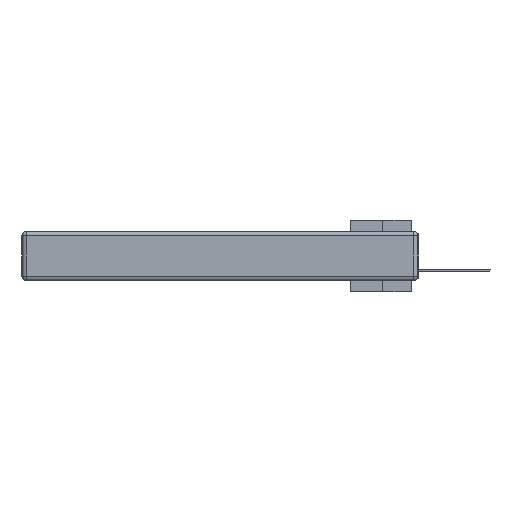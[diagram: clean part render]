
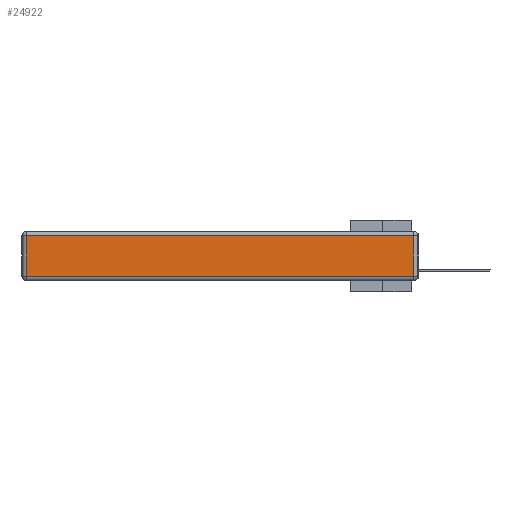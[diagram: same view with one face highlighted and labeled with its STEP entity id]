
A CAD part, left-side view. The second image highlights one B-rep face of the part: STEP entity #24922.
In plain terms, the highlighted planar face has unit normal (-1, 0, 0).
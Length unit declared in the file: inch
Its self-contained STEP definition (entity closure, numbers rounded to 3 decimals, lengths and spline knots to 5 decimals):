
#3186 = VERTEX_POINT ( 'NONE', #13487 ) ;
#3708 = DIRECTION ( 'NONE',  ( 0., 0., 1. ) ) ;
#5612 = EDGE_CURVE ( 'NONE', #34793, #3186, #30370, .T. ) ;
#5786 = EDGE_CURVE ( 'NONE', #8883, #22546, #15652, .T. ) ;
#5871 = CARTESIAN_POINT ( 'NONE',  ( 0., 2.72, -0.313 ) ) ;
#8045 = CARTESIAN_POINT ( 'NONE',  ( 0., 2.75, -0.03 ) ) ;
#8883 = VERTEX_POINT ( 'NONE', #5871 ) ;
#9691 = LINE ( 'NONE', #19569, #11995 ) ;
#11995 = VECTOR ( 'NONE', #25467, 39.37008 ) ;
#12415 = CARTESIAN_POINT ( 'NONE',  ( 0., 0., -0.343 ) ) ;
#13423 = FACE_OUTER_BOUND ( 'NONE', #18129, .T. ) ;
#13487 = CARTESIAN_POINT ( 'NONE',  ( 0., 2.72, -0.03 ) ) ;
#13542 = ORIENTED_EDGE ( 'NONE', *, *, #23218, .T. ) ;
#14140 = ORIENTED_EDGE ( 'NONE', *, *, #5786, .T. ) ;
#14721 = DIRECTION ( 'NONE',  ( 0., -1., 0. ) ) ;
#15652 = LINE ( 'NONE', #29110, #27167 ) ;
#18129 = EDGE_LOOP ( 'NONE', ( #14140, #28127, #31392, #13542 ) ) ;
#18329 = DIRECTION ( 'NONE',  ( -1., 0., 0. ) ) ;
#19569 = CARTESIAN_POINT ( 'NONE',  ( 0., 0.03, -0.343 ) ) ;
#21545 = CARTESIAN_POINT ( 'NONE',  ( 0., 0.03, -0.313 ) ) ;
#21897 = DIRECTION ( 'NONE',  ( 0., 0., -1. ) ) ;
#22546 = VERTEX_POINT ( 'NONE', #21545 ) ;
#23218 = EDGE_CURVE ( 'NONE', #3186, #8883, #34730, .T. ) ;
#24922 = ADVANCED_FACE ( 'NONE', ( #13423 ), #30014, .T. ) ;
#25467 = DIRECTION ( 'NONE',  ( 0., 0., 1. ) ) ;
#25581 = EDGE_CURVE ( 'NONE', #22546, #34793, #9691, .T. ) ;
#26305 = CARTESIAN_POINT ( 'NONE',  ( 0., 0.03, -0.03 ) ) ;
#26621 = AXIS2_PLACEMENT_3D ( 'NONE', #12415, #18329, #3708 ) ;
#27167 = VECTOR ( 'NONE', #14721, 39.37008 ) ;
#28127 = ORIENTED_EDGE ( 'NONE', *, *, #25581, .T. ) ;
#29110 = CARTESIAN_POINT ( 'NONE',  ( 0., 0., -0.313 ) ) ;
#30014 = PLANE ( 'NONE',  #26621 ) ;
#30370 = LINE ( 'NONE', #8045, #37245 ) ;
#31392 = ORIENTED_EDGE ( 'NONE', *, *, #5612, .T. ) ;
#33802 = VECTOR ( 'NONE', #21897, 39.37008 ) ;
#34730 = LINE ( 'NONE', #37036, #33802 ) ;
#34793 = VERTEX_POINT ( 'NONE', #26305 ) ;
#37036 = CARTESIAN_POINT ( 'NONE',  ( 0., 2.72, -0.343 ) ) ;
#37245 = VECTOR ( 'NONE', #37834, 39.37008 ) ;
#37834 = DIRECTION ( 'NONE',  ( 0., 1., 0. ) ) ;
